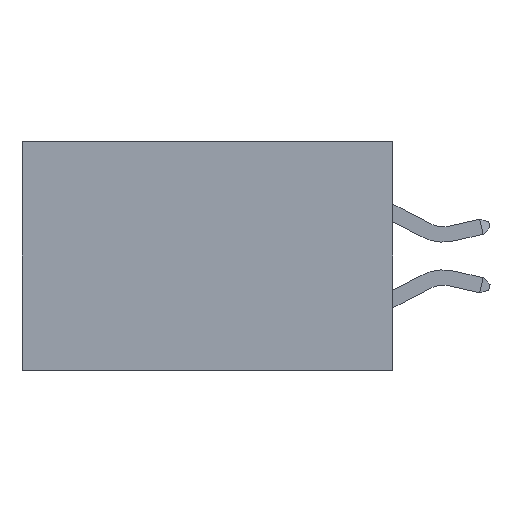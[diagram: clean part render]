
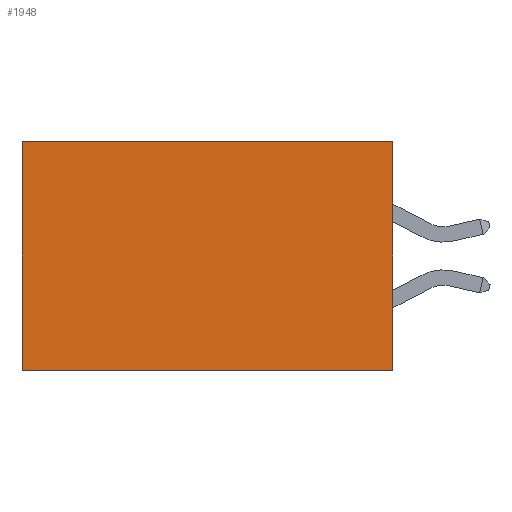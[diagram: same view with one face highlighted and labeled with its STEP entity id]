
A CAD part, left-side view. The second image highlights one B-rep face of the part: STEP entity #1948.
In plain terms, the highlighted planar face has unit normal (-1, 0, 0).
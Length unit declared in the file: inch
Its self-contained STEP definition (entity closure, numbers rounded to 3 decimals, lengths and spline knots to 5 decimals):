
#1803 = PLANE ( 'NONE',  #14098 ) ;
#1948 = ADVANCED_FACE ( 'NONE', ( #12716 ), #1803, .F. ) ;
#2181 = CARTESIAN_POINT ( 'NONE',  ( 0.2875, 0., 0. ) ) ;
#2839 = LINE ( 'NONE', #15527, #19229 ) ;
#4470 = CARTESIAN_POINT ( 'NONE',  ( 0.2875, 0.6, 0. ) ) ;
#4529 = LINE ( 'NONE', #12788, #10239 ) ;
#4723 = DIRECTION ( 'NONE',  ( 0., 0., -1. ) ) ;
#5219 = CARTESIAN_POINT ( 'NONE',  ( 0.2875, 0., 0. ) ) ;
#5635 = ORIENTED_EDGE ( 'NONE', *, *, #10793, .T. ) ;
#5772 = ORIENTED_EDGE ( 'NONE', *, *, #20059, .F. ) ;
#6411 = EDGE_CURVE ( 'NONE', #15150, #15740, #2839, .T. ) ;
#6771 = CARTESIAN_POINT ( 'NONE',  ( 0.2875, 0., -0.37 ) ) ;
#7234 = ORIENTED_EDGE ( 'NONE', *, *, #13607, .F. ) ;
#10239 = VECTOR ( 'NONE', #4723, 39.37008 ) ;
#10793 = EDGE_CURVE ( 'NONE', #15740, #15148, #4529, .T. ) ;
#11497 = VECTOR ( 'NONE', #15132, 39.37008 ) ;
#11530 = EDGE_LOOP ( 'NONE', ( #5635, #5772, #7234, #14536 ) ) ;
#11704 = CARTESIAN_POINT ( 'NONE',  ( 0.2875, 0.6, -0.37 ) ) ;
#12716 = FACE_OUTER_BOUND ( 'NONE', #11530, .T. ) ;
#12788 = CARTESIAN_POINT ( 'NONE',  ( 0.2875, 0.6, 0. ) ) ;
#13607 = EDGE_CURVE ( 'NONE', #15150, #19321, #18021, .T. ) ;
#14098 = AXIS2_PLACEMENT_3D ( 'NONE', #14520, #14920, #17908 ) ;
#14520 = CARTESIAN_POINT ( 'NONE',  ( 0.2875, 0., 0. ) ) ;
#14536 = ORIENTED_EDGE ( 'NONE', *, *, #6411, .T. ) ;
#14920 = DIRECTION ( 'NONE',  ( 1., 0., 0. ) ) ;
#15132 = DIRECTION ( 'NONE',  ( 0., 1., 0. ) ) ;
#15148 = VERTEX_POINT ( 'NONE', #11704 ) ;
#15150 = VERTEX_POINT ( 'NONE', #2181 ) ;
#15527 = CARTESIAN_POINT ( 'NONE',  ( 0.2875, 0., 0. ) ) ;
#15740 = VERTEX_POINT ( 'NONE', #4470 ) ;
#16924 = DIRECTION ( 'NONE',  ( 0., 0., -1. ) ) ;
#17908 = DIRECTION ( 'NONE',  ( 0., 0., -1. ) ) ;
#18021 = LINE ( 'NONE', #5219, #18516 ) ;
#18348 = CARTESIAN_POINT ( 'NONE',  ( 0.2875, 0., -0.37 ) ) ;
#18516 = VECTOR ( 'NONE', #16924, 39.37008 ) ;
#19229 = VECTOR ( 'NONE', #20340, 39.37008 ) ;
#19321 = VERTEX_POINT ( 'NONE', #6771 ) ;
#19954 = LINE ( 'NONE', #18348, #11497 ) ;
#20059 = EDGE_CURVE ( 'NONE', #19321, #15148, #19954, .T. ) ;
#20340 = DIRECTION ( 'NONE',  ( 0., 1., 0. ) ) ;
